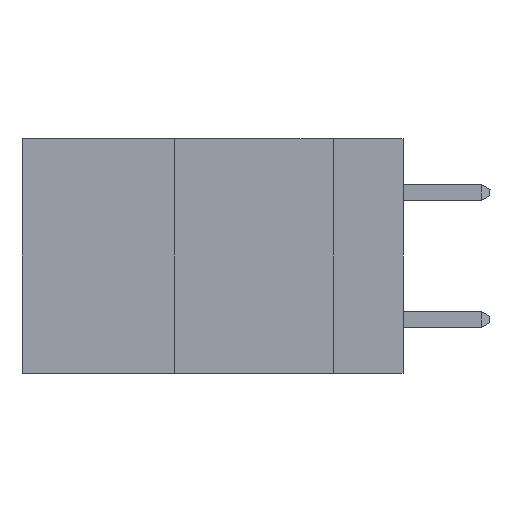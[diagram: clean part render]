
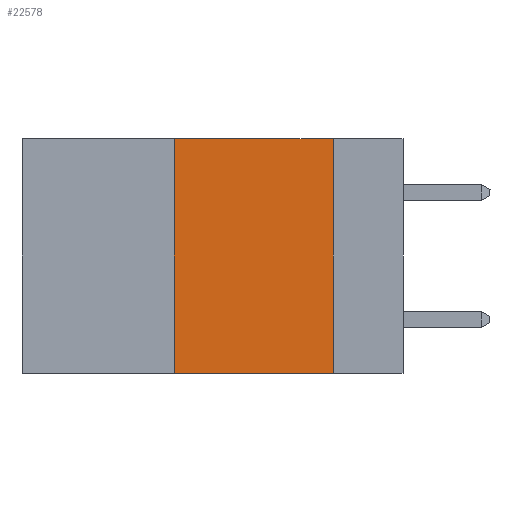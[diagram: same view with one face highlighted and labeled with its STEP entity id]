
A CAD part, left-side view. The second image highlights one B-rep face of the part: STEP entity #22578.
In plain terms, the highlighted planar face has unit normal (-1, 0, 0).
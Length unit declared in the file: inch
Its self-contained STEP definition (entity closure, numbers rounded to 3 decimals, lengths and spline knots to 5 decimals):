
#197 = EDGE_LOOP ( 'NONE', ( #38038, #32887, #36330, #27747 ) ) ;
#849 = EDGE_CURVE ( 'NONE', #13159, #10107, #24568, .T. ) ;
#1582 = LINE ( 'NONE', #40229, #39362 ) ;
#1624 = LINE ( 'NONE', #26330, #29638 ) ;
#1802 = LINE ( 'NONE', #28534, #20118 ) ;
#2991 = DIRECTION ( 'NONE',  ( 0., 0., -1. ) ) ;
#4448 = DIRECTION ( 'NONE',  ( 0., 0., 1. ) ) ;
#10107 = VERTEX_POINT ( 'NONE', #13291 ) ;
#11012 = VERTEX_POINT ( 'NONE', #14487 ) ;
#13159 = VERTEX_POINT ( 'NONE', #30293 ) ;
#13291 = CARTESIAN_POINT ( 'NONE',  ( 0., 0.36, 0. ) ) ;
#14487 = CARTESIAN_POINT ( 'NONE',  ( 0., 0.11, 0. ) ) ;
#15320 = CARTESIAN_POINT ( 'NONE',  ( 0., 0.36, 0. ) ) ;
#17555 = PLANE ( 'NONE',  #43899 ) ;
#20118 = VECTOR ( 'NONE', #25017, 39.37008 ) ;
#22076 = FACE_OUTER_BOUND ( 'NONE', #197, .T. ) ;
#22578 = ADVANCED_FACE ( 'NONE', ( #22076 ), #17555, .F. ) ;
#24568 = LINE ( 'NONE', #15320, #42879 ) ;
#24884 = DIRECTION ( 'NONE',  ( 1., 0., 0. ) ) ;
#25017 = DIRECTION ( 'NONE',  ( 0., -1., 0. ) ) ;
#26330 = CARTESIAN_POINT ( 'NONE',  ( 0., 0.11, 0. ) ) ;
#27205 = VERTEX_POINT ( 'NONE', #46379 ) ;
#27747 = ORIENTED_EDGE ( 'NONE', *, *, #28719, .T. ) ;
#28288 = EDGE_CURVE ( 'NONE', #11012, #27205, #1624, .T. ) ;
#28405 = CARTESIAN_POINT ( 'NONE',  ( 0., 0.6, 0. ) ) ;
#28534 = CARTESIAN_POINT ( 'NONE',  ( 0., 0.6, 0. ) ) ;
#28719 = EDGE_CURVE ( 'NONE', #13159, #27205, #1582, .T. ) ;
#29638 = VECTOR ( 'NONE', #30008, 39.37008 ) ;
#30008 = DIRECTION ( 'NONE',  ( 0., 0., -1. ) ) ;
#30293 = CARTESIAN_POINT ( 'NONE',  ( 0., 0.36, -0.37 ) ) ;
#32887 = ORIENTED_EDGE ( 'NONE', *, *, #46942, .F. ) ;
#36330 = ORIENTED_EDGE ( 'NONE', *, *, #849, .F. ) ;
#36711 = DIRECTION ( 'NONE',  ( 0., -1., 0. ) ) ;
#38038 = ORIENTED_EDGE ( 'NONE', *, *, #28288, .F. ) ;
#39362 = VECTOR ( 'NONE', #36711, 39.37008 ) ;
#40229 = CARTESIAN_POINT ( 'NONE',  ( 0., 0.6, -0.37 ) ) ;
#42879 = VECTOR ( 'NONE', #4448, 39.37008 ) ;
#43899 = AXIS2_PLACEMENT_3D ( 'NONE', #28405, #24884, #2991 ) ;
#46379 = CARTESIAN_POINT ( 'NONE',  ( 0., 0.11, -0.37 ) ) ;
#46942 = EDGE_CURVE ( 'NONE', #10107, #11012, #1802, .T. ) ;
